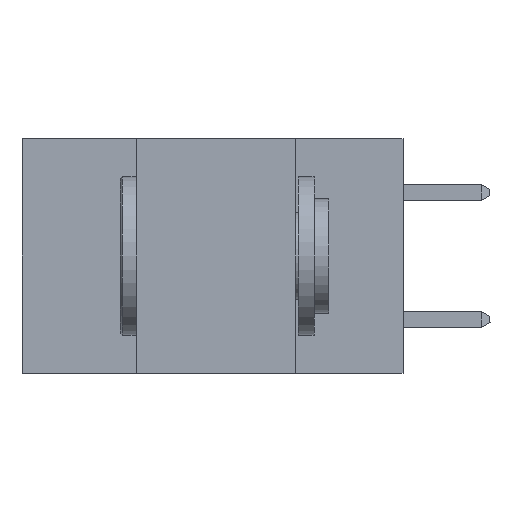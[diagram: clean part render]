
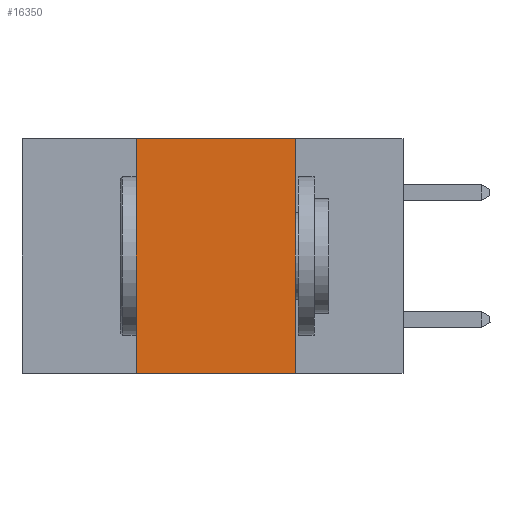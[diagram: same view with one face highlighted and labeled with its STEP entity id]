
A CAD part, left-side view. The second image highlights one B-rep face of the part: STEP entity #16350.
In plain terms, the highlighted planar face has unit normal (-1, 0, 0).
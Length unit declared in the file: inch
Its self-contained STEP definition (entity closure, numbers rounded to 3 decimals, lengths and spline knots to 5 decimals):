
#567 = CARTESIAN_POINT ( 'NONE',  ( 0., 0.17, 0. ) ) ;
#2561 = CARTESIAN_POINT ( 'NONE',  ( 0., 0.6, 0. ) ) ;
#3545 = EDGE_CURVE ( 'NONE', #13621, #7969, #37116, .T. ) ;
#5283 = VECTOR ( 'NONE', #15063, 39.37008 ) ;
#5358 = PLANE ( 'NONE',  #14476 ) ;
#5418 = EDGE_CURVE ( 'NONE', #8507, #5470, #17958, .T. ) ;
#5470 = VERTEX_POINT ( 'NONE', #13463 ) ;
#7011 = LINE ( 'NONE', #30890, #35149 ) ;
#7969 = VERTEX_POINT ( 'NONE', #567 ) ;
#8507 = VERTEX_POINT ( 'NONE', #10587 ) ;
#9245 = ORIENTED_EDGE ( 'NONE', *, *, #3545, .F. ) ;
#10587 = CARTESIAN_POINT ( 'NONE',  ( 0., 0.42, -0.37 ) ) ;
#10745 = ORIENTED_EDGE ( 'NONE', *, *, #5418, .T. ) ;
#13463 = CARTESIAN_POINT ( 'NONE',  ( 0., 0.17, -0.37 ) ) ;
#13621 = VERTEX_POINT ( 'NONE', #31455 ) ;
#14476 = AXIS2_PLACEMENT_3D ( 'NONE', #2561, #22963, #15391 ) ;
#15063 = DIRECTION ( 'NONE',  ( 0., -1., 0. ) ) ;
#15391 = DIRECTION ( 'NONE',  ( 0., 0., -1. ) ) ;
#16175 = DIRECTION ( 'NONE',  ( 0., 0., -1. ) ) ;
#16350 = ADVANCED_FACE ( 'NONE', ( #32332 ), #5358, .F. ) ;
#17958 = LINE ( 'NONE', #33284, #28441 ) ;
#21432 = CARTESIAN_POINT ( 'NONE',  ( 0., 0.42, 0. ) ) ;
#22963 = DIRECTION ( 'NONE',  ( 1., 0., 0. ) ) ;
#23515 = CARTESIAN_POINT ( 'NONE',  ( 0., 0.6, 0. ) ) ;
#23562 = EDGE_LOOP ( 'NONE', ( #30248, #9245, #24539, #10745 ) ) ;
#23604 = LINE ( 'NONE', #21432, #33502 ) ;
#24539 = ORIENTED_EDGE ( 'NONE', *, *, #25890, .F. ) ;
#25890 = EDGE_CURVE ( 'NONE', #8507, #13621, #23604, .T. ) ;
#27621 = DIRECTION ( 'NONE',  ( 0., 0., 1. ) ) ;
#28441 = VECTOR ( 'NONE', #36244, 39.37008 ) ;
#29394 = EDGE_CURVE ( 'NONE', #7969, #5470, #7011, .T. ) ;
#30248 = ORIENTED_EDGE ( 'NONE', *, *, #29394, .F. ) ;
#30890 = CARTESIAN_POINT ( 'NONE',  ( 0., 0.17, 0. ) ) ;
#31455 = CARTESIAN_POINT ( 'NONE',  ( 0., 0.42, 0. ) ) ;
#32332 = FACE_OUTER_BOUND ( 'NONE', #23562, .T. ) ;
#33284 = CARTESIAN_POINT ( 'NONE',  ( 0., 0.6, -0.37 ) ) ;
#33502 = VECTOR ( 'NONE', #27621, 39.37008 ) ;
#35149 = VECTOR ( 'NONE', #16175, 39.37008 ) ;
#36244 = DIRECTION ( 'NONE',  ( 0., -1., 0. ) ) ;
#37116 = LINE ( 'NONE', #23515, #5283 ) ;
